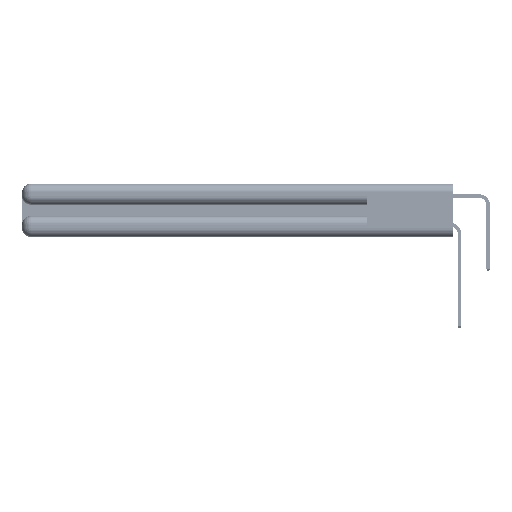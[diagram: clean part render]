
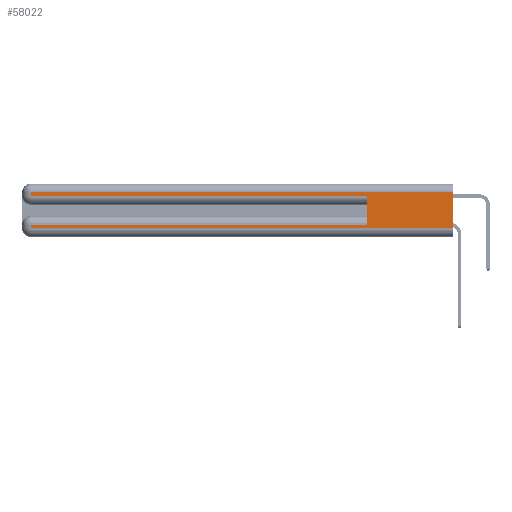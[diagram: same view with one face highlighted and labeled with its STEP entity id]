
A CAD part, left-side view. The second image highlights one B-rep face of the part: STEP entity #58022.
In plain terms, the highlighted planar face has unit normal (-1, 0, 0).
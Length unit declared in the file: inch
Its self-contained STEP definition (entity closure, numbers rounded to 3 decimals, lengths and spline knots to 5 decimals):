
#4174 = CARTESIAN_POINT ( 'NONE',  ( 0., 0., 0.06 ) ) ;
#5780 = EDGE_CURVE ( 'NONE', #19128, #26035, #18653, .T. ) ;
#5896 = DIRECTION ( 'NONE',  ( 0., 1., 0. ) ) ;
#5966 = DIRECTION ( 'NONE',  ( 0., -1., 0. ) ) ;
#6419 = ORIENTED_EDGE ( 'NONE', *, *, #32001, .T. ) ;
#6848 = CARTESIAN_POINT ( 'NONE',  ( 0., 2.94, 0.285 ) ) ;
#7192 = DIRECTION ( 'NONE',  ( 0., 0., -1. ) ) ;
#8502 = ORIENTED_EDGE ( 'NONE', *, *, #48216, .F. ) ;
#8522 = DIRECTION ( 'NONE',  ( 1., 0., 0. ) ) ;
#8621 = AXIS2_PLACEMENT_3D ( 'NONE', #35473, #8522, #40230 ) ;
#8782 = DIRECTION ( 'NONE',  ( 0., -1., 0. ) ) ;
#11141 = FACE_OUTER_BOUND ( 'NONE', #32320, .T. ) ;
#13066 = VERTEX_POINT ( 'NONE', #19144 ) ;
#13708 = EDGE_CURVE ( 'NONE', #50045, #55707, #33756, .T. ) ;
#16263 = DIRECTION ( 'NONE',  ( 0., 0., -1. ) ) ;
#16377 = VECTOR ( 'NONE', #47786, 39.37008 ) ;
#16845 = CARTESIAN_POINT ( 'NONE',  ( 0., 2.94, 0.06 ) ) ;
#17609 = EDGE_CURVE ( 'NONE', #26035, #48968, #48862, .T. ) ;
#17826 = CARTESIAN_POINT ( 'NONE',  ( 0., 0., 0.37 ) ) ;
#18653 = LINE ( 'NONE', #33081, #20081 ) ;
#19128 = VERTEX_POINT ( 'NONE', #25597 ) ;
#19144 = CARTESIAN_POINT ( 'NONE',  ( 0., 2.94, 0.31 ) ) ;
#20081 = VECTOR ( 'NONE', #5896, 39.37008 ) ;
#20474 = LINE ( 'NONE', #34355, #33937 ) ;
#21951 = ORIENTED_EDGE ( 'NONE', *, *, #13708, .T. ) ;
#22422 = DIRECTION ( 'NONE',  ( 0., 0., -1. ) ) ;
#24513 = CARTESIAN_POINT ( 'NONE',  ( 0., 0., 0.31 ) ) ;
#25268 = CARTESIAN_POINT ( 'NONE',  ( 0., 0.6, 0.145 ) ) ;
#25597 = CARTESIAN_POINT ( 'NONE',  ( 0., 0.6, 0.085 ) ) ;
#26035 = VERTEX_POINT ( 'NONE', #50824 ) ;
#26319 = VERTEX_POINT ( 'NONE', #52545 ) ;
#27716 = VECTOR ( 'NONE', #16263, 39.37008 ) ;
#29898 = LINE ( 'NONE', #25268, #16377 ) ;
#30941 = VECTOR ( 'NONE', #5966, 39.37008 ) ;
#32001 = EDGE_CURVE ( 'NONE', #13066, #50045, #20474, .T. ) ;
#32320 = EDGE_LOOP ( 'NONE', ( #52392, #58054, #6419, #21951, #8502, #36901, #54537, #53849 ) ) ;
#32474 = LINE ( 'NONE', #17826, #43045 ) ;
#33081 = CARTESIAN_POINT ( 'NONE',  ( 0., 0., 0.085 ) ) ;
#33100 = VECTOR ( 'NONE', #41087, 39.37008 ) ;
#33149 = CARTESIAN_POINT ( 'NONE',  ( 0., 0., 0.285 ) ) ;
#33756 = LINE ( 'NONE', #33149, #30941 ) ;
#33876 = EDGE_CURVE ( 'NONE', #49992, #13066, #57065, .T. ) ;
#33937 = VECTOR ( 'NONE', #7192, 39.37008 ) ;
#34355 = CARTESIAN_POINT ( 'NONE',  ( 0., 2.94, 0.37 ) ) ;
#35473 = CARTESIAN_POINT ( 'NONE',  ( 0., 0., 0.37 ) ) ;
#36901 = ORIENTED_EDGE ( 'NONE', *, *, #5780, .T. ) ;
#36937 = VECTOR ( 'NONE', #8782, 39.37008 ) ;
#38358 = LINE ( 'NONE', #4174, #36937 ) ;
#40230 = DIRECTION ( 'NONE',  ( 0., 0., -1. ) ) ;
#41087 = DIRECTION ( 'NONE',  ( 0., 1., 0. ) ) ;
#43045 = VECTOR ( 'NONE', #22422, 39.37008 ) ;
#43402 = CARTESIAN_POINT ( 'NONE',  ( 0., 2.94, 0.37 ) ) ;
#47786 = DIRECTION ( 'NONE',  ( 0., 0., 1. ) ) ;
#48216 = EDGE_CURVE ( 'NONE', #19128, #55707, #29898, .T. ) ;
#48445 = EDGE_CURVE ( 'NONE', #48968, #26319, #38358, .T. ) ;
#48862 = LINE ( 'NONE', #43402, #27716 ) ;
#48968 = VERTEX_POINT ( 'NONE', #16845 ) ;
#49992 = VERTEX_POINT ( 'NONE', #24513 ) ;
#50045 = VERTEX_POINT ( 'NONE', #6848 ) ;
#50824 = CARTESIAN_POINT ( 'NONE',  ( 0., 2.94, 0.085 ) ) ;
#52392 = ORIENTED_EDGE ( 'NONE', *, *, #58064, .F. ) ;
#52545 = CARTESIAN_POINT ( 'NONE',  ( 0., 0., 0.06 ) ) ;
#53849 = ORIENTED_EDGE ( 'NONE', *, *, #48445, .T. ) ;
#54246 = CARTESIAN_POINT ( 'NONE',  ( 0., 0.6, 0.285 ) ) ;
#54537 = ORIENTED_EDGE ( 'NONE', *, *, #17609, .T. ) ;
#54655 = CARTESIAN_POINT ( 'NONE',  ( 0., 0., 0.31 ) ) ;
#55707 = VERTEX_POINT ( 'NONE', #54246 ) ;
#57065 = LINE ( 'NONE', #54655, #33100 ) ;
#58022 = ADVANCED_FACE ( 'NONE', ( #11141 ), #58154, .F. ) ;
#58054 = ORIENTED_EDGE ( 'NONE', *, *, #33876, .T. ) ;
#58064 = EDGE_CURVE ( 'NONE', #49992, #26319, #32474, .T. ) ;
#58154 = PLANE ( 'NONE',  #8621 ) ;
